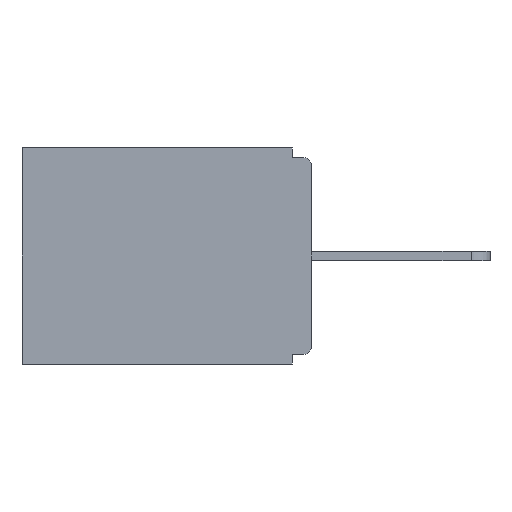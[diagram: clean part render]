
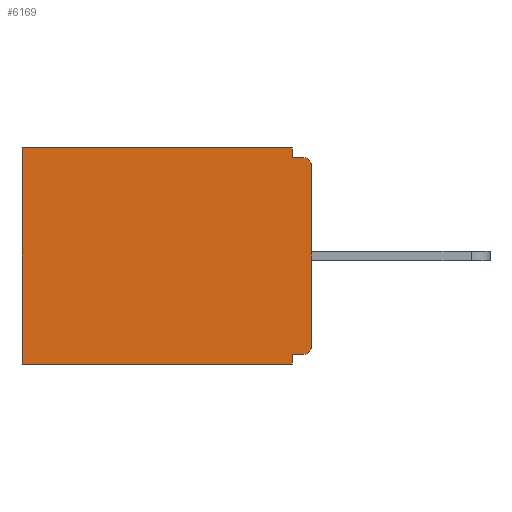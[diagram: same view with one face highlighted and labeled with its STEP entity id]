
A CAD part, left-side view. The second image highlights one B-rep face of the part: STEP entity #6169.
In plain terms, the highlighted planar face has unit normal (-1, 0, 0).
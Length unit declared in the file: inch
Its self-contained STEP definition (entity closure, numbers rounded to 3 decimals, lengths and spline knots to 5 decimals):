
#86 = VERTEX_POINT ( 'NONE', #6879 ) ;
#91 = CARTESIAN_POINT ( 'NONE',  ( 0.298, 0.031, -0.328 ) ) ;
#152 = LINE ( 'NONE', #1266, #5176 ) ;
#174 = EDGE_CURVE ( 'NONE', #86, #2605, #9922, .T. ) ;
#503 = EDGE_CURVE ( 'NONE', #6816, #3001, #974, .T. ) ;
#602 = CARTESIAN_POINT ( 'NONE',  ( 0.298, 0., 0. ) ) ;
#643 = CARTESIAN_POINT ( 'NONE',  ( 0.298, 0.031, -0.343 ) ) ;
#644 = DIRECTION ( 'NONE',  ( 1., 0., 0. ) ) ;
#687 = EDGE_CURVE ( 'NONE', #6139, #9050, #4771, .T. ) ;
#832 = CARTESIAN_POINT ( 'NONE',  ( 0.298, 0.031, -0.343 ) ) ;
#890 = FACE_OUTER_BOUND ( 'NONE', #11098, .T. ) ;
#974 = LINE ( 'NONE', #3409, #5893 ) ;
#1140 = CARTESIAN_POINT ( 'NONE',  ( 0.298, 0., -0.328 ) ) ;
#1236 = EDGE_CURVE ( 'NONE', #2583, #3158, #152, .T. ) ;
#1266 = CARTESIAN_POINT ( 'NONE',  ( 0.298, 0., -0.015 ) ) ;
#1321 = VERTEX_POINT ( 'NONE', #643 ) ;
#1335 = DIRECTION ( 'NONE',  ( 0., 0., -1. ) ) ;
#1471 = EDGE_CURVE ( 'NONE', #6139, #2605, #7682, .T. ) ;
#1547 = VECTOR ( 'NONE', #6721, 39.37008 ) ;
#1637 = VERTEX_POINT ( 'NONE', #3503 ) ;
#1802 = EDGE_CURVE ( 'NONE', #86, #3158, #9006, .T. ) ;
#1894 = LINE ( 'NONE', #8964, #1547 ) ;
#1972 = ORIENTED_EDGE ( 'NONE', *, *, #5006, .F. ) ;
#2371 = CARTESIAN_POINT ( 'NONE',  ( 0.298, 0., 0. ) ) ;
#2377 = ORIENTED_EDGE ( 'NONE', *, *, #174, .F. ) ;
#2583 = VERTEX_POINT ( 'NONE', #4221 ) ;
#2605 = VERTEX_POINT ( 'NONE', #5990 ) ;
#3001 = VERTEX_POINT ( 'NONE', #6554 ) ;
#3158 = VERTEX_POINT ( 'NONE', #3255 ) ;
#3255 = CARTESIAN_POINT ( 'NONE',  ( 0.298, 0.015, -0.015 ) ) ;
#3314 = AXIS2_PLACEMENT_3D ( 'NONE', #5357, #644, #9451 ) ;
#3380 = ORIENTED_EDGE ( 'NONE', *, *, #503, .T. ) ;
#3409 = CARTESIAN_POINT ( 'NONE',  ( 0.298, 0.46, 0. ) ) ;
#3479 = VECTOR ( 'NONE', #5882, 39.37008 ) ;
#3503 = CARTESIAN_POINT ( 'NONE',  ( 0.298, 0.031, 0. ) ) ;
#3557 = ORIENTED_EDGE ( 'NONE', *, *, #687, .F. ) ;
#3660 = EDGE_CURVE ( 'NONE', #9050, #1321, #1894, .T. ) ;
#3860 = VECTOR ( 'NONE', #8242, 39.37008 ) ;
#4110 = AXIS2_PLACEMENT_3D ( 'NONE', #5057, #6650, #7219 ) ;
#4134 = CARTESIAN_POINT ( 'NONE',  ( 0.298, 0., -0.343 ) ) ;
#4221 = CARTESIAN_POINT ( 'NONE',  ( 0.298, 0.031, -0.015 ) ) ;
#4379 = EDGE_CURVE ( 'NONE', #1637, #2583, #7904, .T. ) ;
#4474 = ORIENTED_EDGE ( 'NONE', *, *, #9747, .T. ) ;
#4771 = LINE ( 'NONE', #1140, #6313 ) ;
#5006 = EDGE_CURVE ( 'NONE', #1321, #3001, #8346, .T. ) ;
#5057 = CARTESIAN_POINT ( 'NONE',  ( 0.298, 0.015, -0.313 ) ) ;
#5176 = VECTOR ( 'NONE', #5498, 39.37008 ) ;
#5342 = DIRECTION ( 'NONE',  ( 0., 1., 0. ) ) ;
#5346 = VECTOR ( 'NONE', #7510, 39.37008 ) ;
#5357 = CARTESIAN_POINT ( 'NONE',  ( 0.298, 0., 0. ) ) ;
#5394 = PLANE ( 'NONE',  #3314 ) ;
#5498 = DIRECTION ( 'NONE',  ( 0., -1., 0. ) ) ;
#5510 = DIRECTION ( 'NONE',  ( 0., 0., -1. ) ) ;
#5524 = VECTOR ( 'NONE', #1335, 39.37008 ) ;
#5882 = DIRECTION ( 'NONE',  ( 0., 1., 0. ) ) ;
#5893 = VECTOR ( 'NONE', #5510, 39.37008 ) ;
#5990 = CARTESIAN_POINT ( 'NONE',  ( 0.298, 0., -0.313 ) ) ;
#6139 = VERTEX_POINT ( 'NONE', #11082 ) ;
#6169 = ADVANCED_FACE ( 'NONE', ( #890 ), #5394, .F. ) ;
#6313 = VECTOR ( 'NONE', #5342, 39.37008 ) ;
#6331 = LINE ( 'NONE', #602, #3860 ) ;
#6554 = CARTESIAN_POINT ( 'NONE',  ( 0.298, 0.46, -0.343 ) ) ;
#6650 = DIRECTION ( 'NONE',  ( -1., 0., 0. ) ) ;
#6721 = DIRECTION ( 'NONE',  ( 0., 0., -1. ) ) ;
#6816 = VERTEX_POINT ( 'NONE', #9640 ) ;
#6879 = CARTESIAN_POINT ( 'NONE',  ( 0.298, 0., -0.03 ) ) ;
#7219 = DIRECTION ( 'NONE',  ( 0., 0., -1. ) ) ;
#7510 = DIRECTION ( 'NONE',  ( 0., 0., -1. ) ) ;
#7682 = CIRCLE ( 'NONE', #4110, 0.015 ) ;
#7753 = ORIENTED_EDGE ( 'NONE', *, *, #1471, .T. ) ;
#7904 = LINE ( 'NONE', #832, #5524 ) ;
#7947 = ORIENTED_EDGE ( 'NONE', *, *, #3660, .F. ) ;
#8242 = DIRECTION ( 'NONE',  ( 0., 1., 0. ) ) ;
#8346 = LINE ( 'NONE', #4134, #3479 ) ;
#8933 = ORIENTED_EDGE ( 'NONE', *, *, #4379, .F. ) ;
#8964 = CARTESIAN_POINT ( 'NONE',  ( 0.298, 0.031, -0.343 ) ) ;
#9006 = CIRCLE ( 'NONE', #9999, 0.015 ) ;
#9050 = VERTEX_POINT ( 'NONE', #91 ) ;
#9360 = ORIENTED_EDGE ( 'NONE', *, *, #1236, .F. ) ;
#9451 = DIRECTION ( 'NONE',  ( 0., 0., -1. ) ) ;
#9640 = CARTESIAN_POINT ( 'NONE',  ( 0.298, 0.46, 0. ) ) ;
#9747 = EDGE_CURVE ( 'NONE', #1637, #6816, #6331, .T. ) ;
#9881 = DIRECTION ( 'NONE',  ( -1., 0., 0. ) ) ;
#9890 = DIRECTION ( 'NONE',  ( 0., 0., -1. ) ) ;
#9922 = LINE ( 'NONE', #2371, #5346 ) ;
#9999 = AXIS2_PLACEMENT_3D ( 'NONE', #10706, #9881, #9890 ) ;
#10005 = ORIENTED_EDGE ( 'NONE', *, *, #1802, .T. ) ;
#10706 = CARTESIAN_POINT ( 'NONE',  ( 0.298, 0.015, -0.03 ) ) ;
#11082 = CARTESIAN_POINT ( 'NONE',  ( 0.298, 0.015, -0.328 ) ) ;
#11098 = EDGE_LOOP ( 'NONE', ( #10005, #9360, #8933, #4474, #3380, #1972, #7947, #3557, #7753, #2377 ) ) ;
